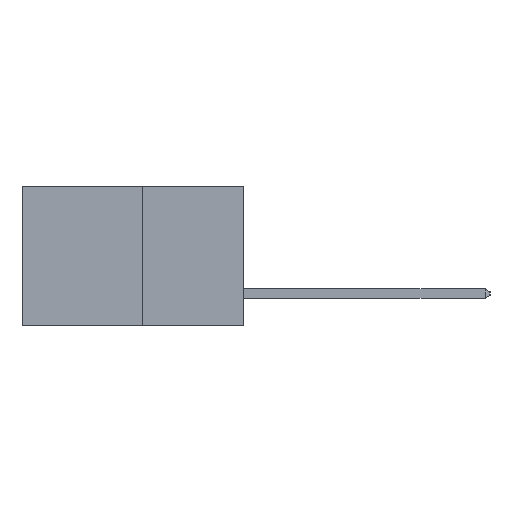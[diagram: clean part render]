
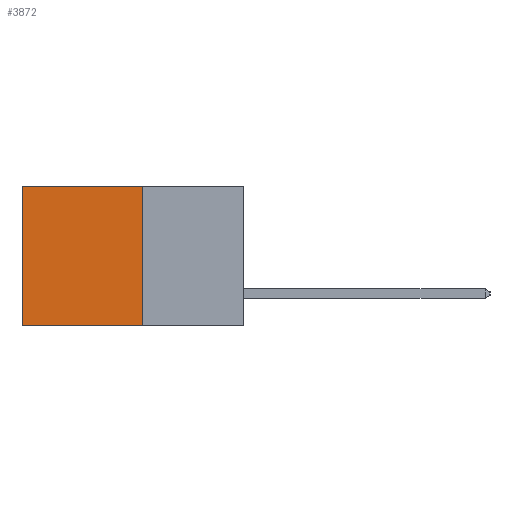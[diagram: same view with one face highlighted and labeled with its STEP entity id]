
A CAD part, left-side view. The second image highlights one B-rep face of the part: STEP entity #3872.
In plain terms, the highlighted planar face has unit normal (-1, 0, 0).
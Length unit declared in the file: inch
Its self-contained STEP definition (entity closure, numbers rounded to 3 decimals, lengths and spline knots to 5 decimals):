
#465 = EDGE_CURVE ( 'NONE', #7871, #5766, #12565, .T. ) ;
#503 = ORIENTED_EDGE ( 'NONE', *, *, #15869, .T. ) ;
#558 = CARTESIAN_POINT ( 'NONE',  ( 0.277, 0.27, -0.37 ) ) ;
#2665 = CARTESIAN_POINT ( 'NONE',  ( 0.277, 0.27, 0. ) ) ;
#3597 = ORIENTED_EDGE ( 'NONE', *, *, #3766, .T. ) ;
#3766 = EDGE_CURVE ( 'NONE', #10293, #4292, #5760, .T. ) ;
#3872 = ADVANCED_FACE ( 'NONE', ( #18437 ), #6364, .F. ) ;
#4292 = VERTEX_POINT ( 'NONE', #12857 ) ;
#4988 = VECTOR ( 'NONE', #5828, 39.37008 ) ;
#5760 = LINE ( 'NONE', #11646, #17385 ) ;
#5766 = VERTEX_POINT ( 'NONE', #13230 ) ;
#5828 = DIRECTION ( 'NONE',  ( 0., 0., -1. ) ) ;
#6043 = LINE ( 'NONE', #11575, #16800 ) ;
#6364 = PLANE ( 'NONE',  #16154 ) ;
#6697 = DIRECTION ( 'NONE',  ( 0., 0., -1. ) ) ;
#6735 = DIRECTION ( 'NONE',  ( 1., 0., 0. ) ) ;
#6889 = DIRECTION ( 'NONE',  ( 0., 0., -1. ) ) ;
#7127 = DIRECTION ( 'NONE',  ( 0., 1., 0. ) ) ;
#7507 = ORIENTED_EDGE ( 'NONE', *, *, #15277, .F. ) ;
#7871 = VERTEX_POINT ( 'NONE', #12878 ) ;
#9286 = EDGE_LOOP ( 'NONE', ( #3597, #7507, #14930, #503 ) ) ;
#10293 = VERTEX_POINT ( 'NONE', #16774 ) ;
#11575 = CARTESIAN_POINT ( 'NONE',  ( 0.277, 0.27, -0.37 ) ) ;
#11646 = CARTESIAN_POINT ( 'NONE',  ( 0.277, 0.59, -0.37 ) ) ;
#12565 = LINE ( 'NONE', #15850, #4988 ) ;
#12857 = CARTESIAN_POINT ( 'NONE',  ( 0.277, 0.59, -0.37 ) ) ;
#12878 = CARTESIAN_POINT ( 'NONE',  ( 0.277, 0.27, 0. ) ) ;
#12970 = DIRECTION ( 'NONE',  ( 0., 1., 0. ) ) ;
#13230 = CARTESIAN_POINT ( 'NONE',  ( 0.277, 0.27, -0.37 ) ) ;
#13751 = VECTOR ( 'NONE', #7127, 39.37008 ) ;
#14930 = ORIENTED_EDGE ( 'NONE', *, *, #465, .F. ) ;
#15277 = EDGE_CURVE ( 'NONE', #5766, #4292, #6043, .T. ) ;
#15850 = CARTESIAN_POINT ( 'NONE',  ( 0.277, 0.27, -0.37 ) ) ;
#15869 = EDGE_CURVE ( 'NONE', #7871, #10293, #17399, .T. ) ;
#16154 = AXIS2_PLACEMENT_3D ( 'NONE', #558, #6735, #6697 ) ;
#16774 = CARTESIAN_POINT ( 'NONE',  ( 0.277, 0.59, 0. ) ) ;
#16800 = VECTOR ( 'NONE', #12970, 39.37008 ) ;
#17385 = VECTOR ( 'NONE', #6889, 39.37008 ) ;
#17399 = LINE ( 'NONE', #2665, #13751 ) ;
#18437 = FACE_OUTER_BOUND ( 'NONE', #9286, .T. ) ;
